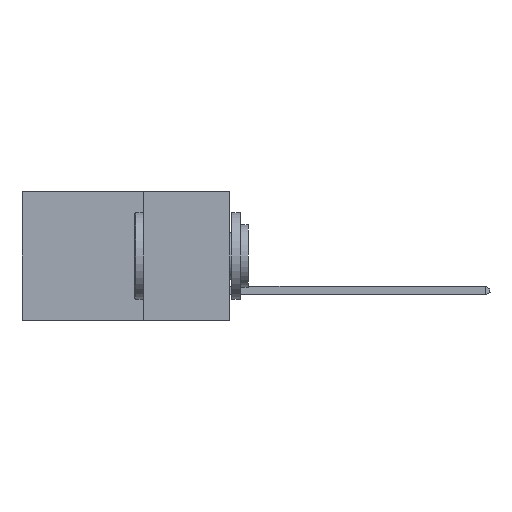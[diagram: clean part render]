
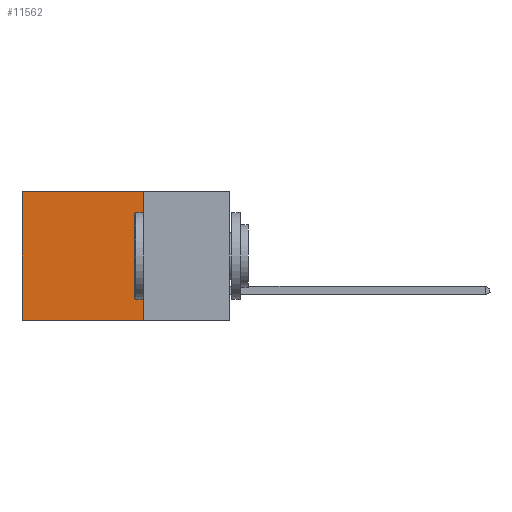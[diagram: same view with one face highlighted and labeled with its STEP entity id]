
A CAD part, left-side view. The second image highlights one B-rep face of the part: STEP entity #11562.
In plain terms, the highlighted planar face has unit normal (-1, 0, 0).
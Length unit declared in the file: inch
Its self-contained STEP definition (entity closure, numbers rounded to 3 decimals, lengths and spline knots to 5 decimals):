
#88 = LINE ( 'NONE', #2311, #4715 ) ;
#992 = LINE ( 'NONE', #4454, #5480 ) ;
#1038 = DIRECTION ( 'NONE',  ( 0., 0., -1. ) ) ;
#1158 = LINE ( 'NONE', #1235, #3333 ) ;
#1235 = CARTESIAN_POINT ( 'NONE',  ( 0.298, 0.25, -0.37 ) ) ;
#1358 = VERTEX_POINT ( 'NONE', #4703 ) ;
#1756 = VERTEX_POINT ( 'NONE', #5253 ) ;
#1931 = DIRECTION ( 'NONE',  ( 1., 0., 0. ) ) ;
#2311 = CARTESIAN_POINT ( 'NONE',  ( 0.298, 0.25, 0. ) ) ;
#2525 = ORIENTED_EDGE ( 'NONE', *, *, #3004, .F. ) ;
#2608 = DIRECTION ( 'NONE',  ( 0., 0., -1. ) ) ;
#2754 = ORIENTED_EDGE ( 'NONE', *, *, #5302, .F. ) ;
#3004 = EDGE_CURVE ( 'NONE', #1358, #1756, #992, .T. ) ;
#3333 = VECTOR ( 'NONE', #9847, 39.37008 ) ;
#4023 = LINE ( 'NONE', #6999, #9846 ) ;
#4454 = CARTESIAN_POINT ( 'NONE',  ( 0.298, 0.25, 0. ) ) ;
#4703 = CARTESIAN_POINT ( 'NONE',  ( 0.298, 0.25, 0. ) ) ;
#4715 = VECTOR ( 'NONE', #10657, 39.37008 ) ;
#5253 = CARTESIAN_POINT ( 'NONE',  ( 0.298, 0.25, -0.37 ) ) ;
#5302 = EDGE_CURVE ( 'NONE', #1756, #5469, #1158, .T. ) ;
#5469 = VERTEX_POINT ( 'NONE', #9509 ) ;
#5480 = VECTOR ( 'NONE', #6330, 39.37008 ) ;
#5537 = ORIENTED_EDGE ( 'NONE', *, *, #10595, .T. ) ;
#6330 = DIRECTION ( 'NONE',  ( 0., 0., -1. ) ) ;
#6559 = CARTESIAN_POINT ( 'NONE',  ( 0.298, 0.25, 0. ) ) ;
#6670 = EDGE_CURVE ( 'NONE', #6713, #5469, #4023, .T. ) ;
#6713 = VERTEX_POINT ( 'NONE', #11161 ) ;
#6999 = CARTESIAN_POINT ( 'NONE',  ( 0.298, 0.6, 0. ) ) ;
#9077 = AXIS2_PLACEMENT_3D ( 'NONE', #6559, #1931, #1038 ) ;
#9469 = PLANE ( 'NONE',  #9077 ) ;
#9509 = CARTESIAN_POINT ( 'NONE',  ( 0.298, 0.6, -0.37 ) ) ;
#9846 = VECTOR ( 'NONE', #2608, 39.37008 ) ;
#9847 = DIRECTION ( 'NONE',  ( 0., 1., 0. ) ) ;
#10366 = FACE_OUTER_BOUND ( 'NONE', #11408, .T. ) ;
#10595 = EDGE_CURVE ( 'NONE', #1358, #6713, #88, .T. ) ;
#10657 = DIRECTION ( 'NONE',  ( 0., 1., 0. ) ) ;
#10764 = ORIENTED_EDGE ( 'NONE', *, *, #6670, .T. ) ;
#11161 = CARTESIAN_POINT ( 'NONE',  ( 0.298, 0.6, 0. ) ) ;
#11408 = EDGE_LOOP ( 'NONE', ( #10764, #2754, #2525, #5537 ) ) ;
#11562 = ADVANCED_FACE ( 'NONE', ( #10366 ), #9469, .F. ) ;
